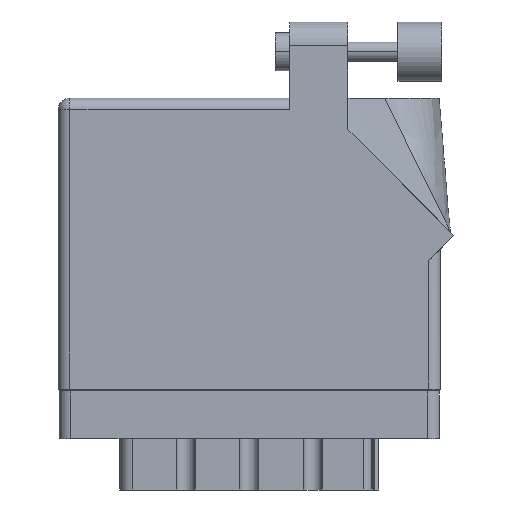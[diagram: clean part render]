
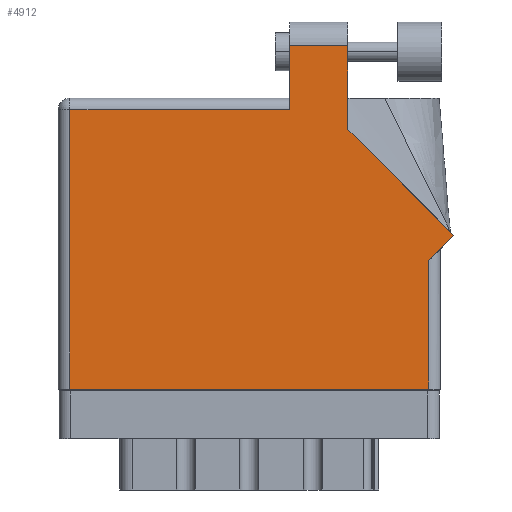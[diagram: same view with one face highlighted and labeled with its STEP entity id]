
A CAD part, front view. The second image highlights one B-rep face of the part: STEP entity #4912.
In plain terms, the highlighted face is planar.
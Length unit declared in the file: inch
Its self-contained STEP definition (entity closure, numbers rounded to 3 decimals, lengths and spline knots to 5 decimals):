
#376 = ORIENTED_EDGE ( 'NONE', *, *, #25013, .T. ) ;
#845 = DIRECTION ( 'NONE',  ( -1., 0., 0. ) ) ;
#1073 = LINE ( 'NONE', #3355, #33407 ) ;
#1588 = CARTESIAN_POINT ( 'NONE',  ( 1.524, 1.36442, 0. ) ) ;
#2472 = LINE ( 'NONE', #33565, #10424 ) ;
#2892 = EDGE_CURVE ( 'NONE', #25518, #34354, #35604, .T. ) ;
#3355 = CARTESIAN_POINT ( 'NONE',  ( 2.01, 0.737, 0. ) ) ;
#4783 = VECTOR ( 'NONE', #22212, 39.37008 ) ;
#4912 = ADVANCED_FACE ( 'NONE', ( #22082 ), #6174, .F. ) ;
#5749 = EDGE_CURVE ( 'NONE', #31731, #26531, #27968, .T. ) ;
#5982 = LINE ( 'NONE', #37777, #28363 ) ;
#6165 = LINE ( 'NONE', #16911, #22070 ) ;
#6174 = PLANE ( 'NONE',  #6367 ) ;
#6367 = AXIS2_PLACEMENT_3D ( 'NONE', #41080, #31214, #8955 ) ;
#7105 = EDGE_CURVE ( 'NONE', #10760, #11510, #18370, .T. ) ;
#7499 = CARTESIAN_POINT ( 'NONE',  ( 1.948, 0.737, 0. ) ) ;
#8098 = ORIENTED_EDGE ( 'NONE', *, *, #40041, .T. ) ;
#8941 = VECTOR ( 'NONE', #9416, 39.37008 ) ;
#8955 = DIRECTION ( 'NONE',  ( -1., 0., 0. ) ) ;
#9416 = DIRECTION ( 'NONE',  ( -0.707, 0.707, 0. ) ) ;
#9961 = ORIENTED_EDGE ( 'NONE', *, *, #5749, .T. ) ;
#10424 = VECTOR ( 'NONE', #36347, 39.37008 ) ;
#10549 = VECTOR ( 'NONE', #845, 39.37008 ) ;
#10760 = VERTEX_POINT ( 'NONE', #28780 ) ;
#10848 = EDGE_CURVE ( 'NONE', #14319, #28768, #6165, .T. ) ;
#11510 = VERTEX_POINT ( 'NONE', #1588 ) ;
#12190 = ORIENTED_EDGE ( 'NONE', *, *, #2892, .T. ) ;
#13018 = CARTESIAN_POINT ( 'NONE',  ( 0.062, 0., 0. ) ) ;
#14296 = DIRECTION ( 'NONE',  ( 0., -1., 0. ) ) ;
#14319 = VERTEX_POINT ( 'NONE', #24310 ) ;
#16421 = VECTOR ( 'NONE', #14296, 39.37008 ) ;
#16911 = CARTESIAN_POINT ( 'NONE',  ( 0., 1.468, 0. ) ) ;
#17152 = EDGE_LOOP ( 'NONE', ( #376, #9961, #36768, #28936, #32513, #12190, #8098, #18395, #18326 ) ) ;
#18326 = ORIENTED_EDGE ( 'NONE', *, *, #7105, .T. ) ;
#18370 = LINE ( 'NONE', #32087, #8941 ) ;
#18395 = ORIENTED_EDGE ( 'NONE', *, *, #36696, .T. ) ;
#19377 = EDGE_CURVE ( 'NONE', #26531, #14319, #5982, .T. ) ;
#22070 = VECTOR ( 'NONE', #38899, 39.37008 ) ;
#22082 = FACE_OUTER_BOUND ( 'NONE', #17152, .T. ) ;
#22212 = DIRECTION ( 'NONE',  ( 1., 0., 0. ) ) ;
#23380 = CARTESIAN_POINT ( 'NONE',  ( 1.217, 1.805, 0. ) ) ;
#23661 = EDGE_CURVE ( 'NONE', #28768, #25518, #40344, .T. ) ;
#24310 = CARTESIAN_POINT ( 'NONE',  ( 1.217, 1.468, 0. ) ) ;
#24724 = DIRECTION ( 'NONE',  ( 0., -1., 0. ) ) ;
#25013 = EDGE_CURVE ( 'NONE', #11510, #31731, #2472, .T. ) ;
#25518 = VERTEX_POINT ( 'NONE', #27776 ) ;
#26531 = VERTEX_POINT ( 'NONE', #23380 ) ;
#27727 = CARTESIAN_POINT ( 'NONE',  ( 1.948, 0., 0. ) ) ;
#27776 = CARTESIAN_POINT ( 'NONE',  ( 0.062, 0., 0. ) ) ;
#27968 = LINE ( 'NONE', #32527, #10549 ) ;
#28030 = CARTESIAN_POINT ( 'NONE',  ( 1.948, 0.675, 0. ) ) ;
#28363 = VECTOR ( 'NONE', #24724, 39.37008 ) ;
#28636 = VECTOR ( 'NONE', #30151, 39.37008 ) ;
#28768 = VERTEX_POINT ( 'NONE', #36213 ) ;
#28780 = CARTESIAN_POINT ( 'NONE',  ( 2.08071, 0.80771, 0. ) ) ;
#28936 = ORIENTED_EDGE ( 'NONE', *, *, #10848, .T. ) ;
#30151 = DIRECTION ( 'NONE',  ( 0., 1., 0. ) ) ;
#31214 = DIRECTION ( 'NONE',  ( 0., 0., -1. ) ) ;
#31731 = VERTEX_POINT ( 'NONE', #36428 ) ;
#32087 = CARTESIAN_POINT ( 'NONE',  ( 2.08071, 0.80771, 0. ) ) ;
#32237 = CARTESIAN_POINT ( 'NONE',  ( 0., 0., 0. ) ) ;
#32513 = ORIENTED_EDGE ( 'NONE', *, *, #23661, .T. ) ;
#32527 = CARTESIAN_POINT ( 'NONE',  ( 1.217, 1.805, 0. ) ) ;
#33407 = VECTOR ( 'NONE', #35446, 39.37008 ) ;
#33565 = CARTESIAN_POINT ( 'NONE',  ( 1.524, 1.36442, 0. ) ) ;
#33780 = VERTEX_POINT ( 'NONE', #28030 ) ;
#34354 = VERTEX_POINT ( 'NONE', #27727 ) ;
#35446 = DIRECTION ( 'NONE',  ( 0.707, 0.707, 0. ) ) ;
#35604 = LINE ( 'NONE', #32237, #4783 ) ;
#36213 = CARTESIAN_POINT ( 'NONE',  ( 0.062, 1.468, 0. ) ) ;
#36347 = DIRECTION ( 'NONE',  ( 0., 1., 0. ) ) ;
#36428 = CARTESIAN_POINT ( 'NONE',  ( 1.524, 1.805, 0. ) ) ;
#36696 = EDGE_CURVE ( 'NONE', #33780, #10760, #1073, .T. ) ;
#36768 = ORIENTED_EDGE ( 'NONE', *, *, #19377, .T. ) ;
#37777 = CARTESIAN_POINT ( 'NONE',  ( 1.217, 1.53, 0. ) ) ;
#38075 = LINE ( 'NONE', #7499, #28636 ) ;
#38899 = DIRECTION ( 'NONE',  ( -1., 0., 0. ) ) ;
#40041 = EDGE_CURVE ( 'NONE', #34354, #33780, #38075, .T. ) ;
#40344 = LINE ( 'NONE', #13018, #16421 ) ;
#41080 = CARTESIAN_POINT ( 'NONE',  ( 0., 1.53, 0. ) ) ;
